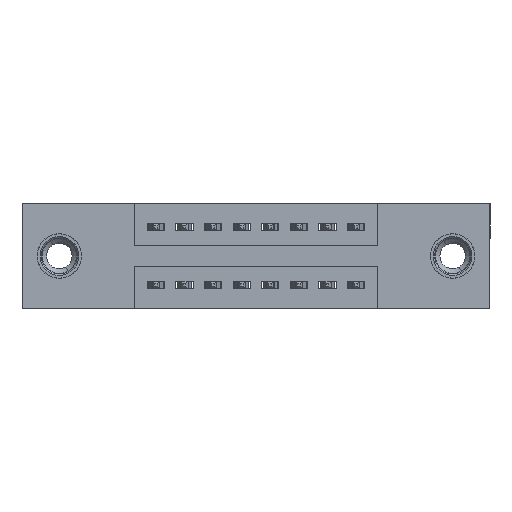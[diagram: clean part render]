
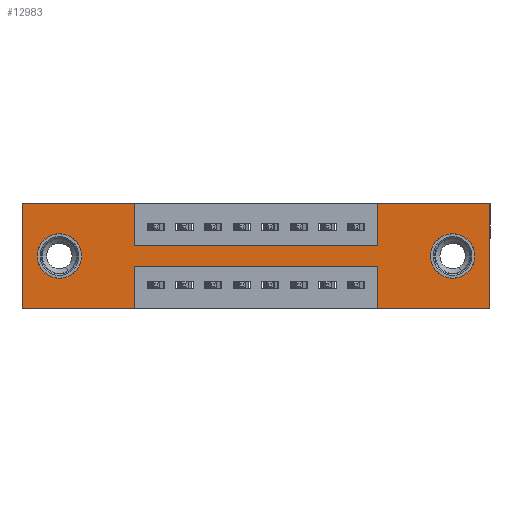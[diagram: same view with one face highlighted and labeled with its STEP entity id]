
A CAD part, front view. The second image highlights one B-rep face of the part: STEP entity #12983.
In plain terms, the highlighted planar face has unit normal (0, -1, 0).
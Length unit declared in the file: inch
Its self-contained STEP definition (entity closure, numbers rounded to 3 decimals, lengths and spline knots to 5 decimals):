
#64 = CARTESIAN_POINT ( 'NONE',  ( 0., 0., 0. ) ) ;
#259 = DIRECTION ( 'NONE',  ( 0., 0., -1. ) ) ;
#395 = VECTOR ( 'NONE', #5062, 39.37008 ) ;
#472 = EDGE_LOOP ( 'NONE', ( #5619, #10605 ) ) ;
#561 = DIRECTION ( 'NONE',  ( 0., 1., 0. ) ) ;
#761 = VERTEX_POINT ( 'NONE', #8621 ) ;
#1044 = CARTESIAN_POINT ( 'NONE',  ( 0.13, 0., -0.107 ) ) ;
#1137 = ORIENTED_EDGE ( 'NONE', *, *, #11477, .F. ) ;
#1145 = ORIENTED_EDGE ( 'NONE', *, *, #5621, .T. ) ;
#1279 = LINE ( 'NONE', #5828, #6372 ) ;
#1359 = EDGE_CURVE ( 'NONE', #10727, #10186, #3395, .T. ) ;
#1416 = VERTEX_POINT ( 'NONE', #9835 ) ;
#1545 = CARTESIAN_POINT ( 'NONE',  ( 1.2425, 0., -0.15 ) ) ;
#1606 = VECTOR ( 'NONE', #2471, 39.37008 ) ;
#1657 = LINE ( 'NONE', #12248, #9697 ) ;
#1683 = AXIS2_PLACEMENT_3D ( 'NONE', #7374, #2345, #9378 ) ;
#1732 = CARTESIAN_POINT ( 'NONE',  ( 0.13, 0., -0.263 ) ) ;
#1822 = CARTESIAN_POINT ( 'NONE',  ( 0., 0., 0. ) ) ;
#1833 = VECTOR ( 'NONE', #11157, 39.37008 ) ;
#1933 = ORIENTED_EDGE ( 'NONE', *, *, #3104, .F. ) ;
#2345 = DIRECTION ( 'NONE',  ( 0., -1., 0. ) ) ;
#2355 = CARTESIAN_POINT ( 'NONE',  ( 1.2425, 0., -0.37 ) ) ;
#2457 = FACE_BOUND ( 'NONE', #6933, .T. ) ;
#2471 = DIRECTION ( 'NONE',  ( -1., 0., 0. ) ) ;
#2588 = ORIENTED_EDGE ( 'NONE', *, *, #7186, .F. ) ;
#2758 = FACE_OUTER_BOUND ( 'NONE', #12592, .T. ) ;
#2913 = CIRCLE ( 'NONE', #12300, 0.078 ) ;
#2937 = CARTESIAN_POINT ( 'NONE',  ( 0.13, 0., -0.185 ) ) ;
#3098 = CIRCLE ( 'NONE', #6126, 0.078 ) ;
#3104 = EDGE_CURVE ( 'NONE', #10186, #7841, #3968, .T. ) ;
#3114 = LINE ( 'NONE', #11016, #395 ) ;
#3244 = LINE ( 'NONE', #5899, #8295 ) ;
#3395 = LINE ( 'NONE', #7033, #8448 ) ;
#3873 = CARTESIAN_POINT ( 'NONE',  ( 1.505, 0., -0.185 ) ) ;
#3944 = DIRECTION ( 'NONE',  ( 0., 0., 1. ) ) ;
#3968 = LINE ( 'NONE', #8499, #1606 ) ;
#4020 = AXIS2_PLACEMENT_3D ( 'NONE', #2937, #9961, #3944 ) ;
#4195 = VECTOR ( 'NONE', #9818, 39.37008 ) ;
#4498 = CARTESIAN_POINT ( 'NONE',  ( 1.2425, 0., -0.22 ) ) ;
#4552 = LINE ( 'NONE', #64, #1833 ) ;
#4839 = DIRECTION ( 'NONE',  ( 0., 0., -1. ) ) ;
#4843 = CARTESIAN_POINT ( 'NONE',  ( 1.635, 0., 0. ) ) ;
#4847 = EDGE_CURVE ( 'NONE', #7894, #5269, #11600, .T. ) ;
#4934 = DIRECTION ( 'NONE',  ( 0., 0., -1. ) ) ;
#5036 = ORIENTED_EDGE ( 'NONE', *, *, #1359, .F. ) ;
#5062 = DIRECTION ( 'NONE',  ( 0., 0., -1. ) ) ;
#5269 = VERTEX_POINT ( 'NONE', #1732 ) ;
#5321 = VERTEX_POINT ( 'NONE', #1822 ) ;
#5619 = ORIENTED_EDGE ( 'NONE', *, *, #4847, .T. ) ;
#5621 = EDGE_CURVE ( 'NONE', #12732, #12567, #8177, .T. ) ;
#5768 = VERTEX_POINT ( 'NONE', #1545 ) ;
#5828 = CARTESIAN_POINT ( 'NONE',  ( 1.2425, 0., -0.37 ) ) ;
#5899 = CARTESIAN_POINT ( 'NONE',  ( 0., 0., 0. ) ) ;
#6044 = CARTESIAN_POINT ( 'NONE',  ( 1.2425, 0., 0. ) ) ;
#6126 = AXIS2_PLACEMENT_3D ( 'NONE', #6665, #561, #7662 ) ;
#6150 = EDGE_CURVE ( 'NONE', #7841, #5321, #4552, .T. ) ;
#6295 = DIRECTION ( 'NONE',  ( -1., 0., 0. ) ) ;
#6366 = DIRECTION ( 'NONE',  ( 0., 1., 0. ) ) ;
#6372 = VECTOR ( 'NONE', #7821, 39.37008 ) ;
#6382 = DIRECTION ( 'NONE',  ( 1., 0., 0. ) ) ;
#6396 = PLANE ( 'NONE',  #1683 ) ;
#6408 = EDGE_CURVE ( 'NONE', #761, #6815, #6458, .T. ) ;
#6458 = LINE ( 'NONE', #10538, #9090 ) ;
#6665 = CARTESIAN_POINT ( 'NONE',  ( 0.13, 0., -0.185 ) ) ;
#6815 = VERTEX_POINT ( 'NONE', #9202 ) ;
#6849 = EDGE_CURVE ( 'NONE', #11630, #8073, #1657, .T. ) ;
#6909 = VECTOR ( 'NONE', #9994, 39.37008 ) ;
#6933 = EDGE_LOOP ( 'NONE', ( #1145, #11306 ) ) ;
#7017 = CARTESIAN_POINT ( 'NONE',  ( 0.3925, 0., -0.22 ) ) ;
#7033 = CARTESIAN_POINT ( 'NONE',  ( 0.3925, 0., -0.37 ) ) ;
#7034 = DIRECTION ( 'NONE',  ( 0., 0., 1. ) ) ;
#7096 = LINE ( 'NONE', #9367, #12402 ) ;
#7186 = EDGE_CURVE ( 'NONE', #5321, #761, #3244, .T. ) ;
#7221 = LINE ( 'NONE', #7017, #6909 ) ;
#7374 = CARTESIAN_POINT ( 'NONE',  ( 0., 0., -0.37 ) ) ;
#7441 = VECTOR ( 'NONE', #7034, 39.37008 ) ;
#7662 = DIRECTION ( 'NONE',  ( 0., 0., 1. ) ) ;
#7667 = ORIENTED_EDGE ( 'NONE', *, *, #11609, .F. ) ;
#7714 = CARTESIAN_POINT ( 'NONE',  ( 0.3925, 0., -0.22 ) ) ;
#7734 = ORIENTED_EDGE ( 'NONE', *, *, #12108, .F. ) ;
#7737 = CARTESIAN_POINT ( 'NONE',  ( 1.505, 0., -0.263 ) ) ;
#7821 = DIRECTION ( 'NONE',  ( 0., 0., 1. ) ) ;
#7841 = VERTEX_POINT ( 'NONE', #9979 ) ;
#7894 = VERTEX_POINT ( 'NONE', #1044 ) ;
#7903 = ORIENTED_EDGE ( 'NONE', *, *, #6408, .F. ) ;
#8016 = CARTESIAN_POINT ( 'NONE',  ( 1.635, 0., -0.37 ) ) ;
#8073 = VERTEX_POINT ( 'NONE', #2355 ) ;
#8177 = CIRCLE ( 'NONE', #10905, 0.078 ) ;
#8295 = VECTOR ( 'NONE', #10808, 39.37008 ) ;
#8448 = VECTOR ( 'NONE', #4839, 39.37008 ) ;
#8499 = CARTESIAN_POINT ( 'NONE',  ( 0., 0., -0.37 ) ) ;
#8560 = DIRECTION ( 'NONE',  ( 0., 0., -1. ) ) ;
#8621 = CARTESIAN_POINT ( 'NONE',  ( 0.3925, 0., 0. ) ) ;
#9090 = VECTOR ( 'NONE', #8560, 39.37008 ) ;
#9202 = CARTESIAN_POINT ( 'NONE',  ( 0.3925, 0., -0.15 ) ) ;
#9367 = CARTESIAN_POINT ( 'NONE',  ( 0.3925, 0., -0.15 ) ) ;
#9378 = DIRECTION ( 'NONE',  ( 0., 0., -1. ) ) ;
#9555 = EDGE_CURVE ( 'NONE', #8073, #11880, #1279, .T. ) ;
#9697 = VECTOR ( 'NONE', #6295, 39.37008 ) ;
#9705 = EDGE_CURVE ( 'NONE', #5768, #1416, #12741, .T. ) ;
#9747 = ORIENTED_EDGE ( 'NONE', *, *, #10442, .F. ) ;
#9782 = CARTESIAN_POINT ( 'NONE',  ( 0., 0., 0. ) ) ;
#9818 = DIRECTION ( 'NONE',  ( 1., 0., 0. ) ) ;
#9835 = CARTESIAN_POINT ( 'NONE',  ( 1.2425, 0., 0. ) ) ;
#9961 = DIRECTION ( 'NONE',  ( 0., 1., 0. ) ) ;
#9979 = CARTESIAN_POINT ( 'NONE',  ( 0., 0., -0.37 ) ) ;
#9994 = DIRECTION ( 'NONE',  ( -1., 0., 0. ) ) ;
#10186 = VERTEX_POINT ( 'NONE', #10913 ) ;
#10364 = ORIENTED_EDGE ( 'NONE', *, *, #6150, .F. ) ;
#10442 = EDGE_CURVE ( 'NONE', #6815, #5768, #7096, .T. ) ;
#10538 = CARTESIAN_POINT ( 'NONE',  ( 0.3925, 0., 0. ) ) ;
#10605 = ORIENTED_EDGE ( 'NONE', *, *, #11965, .T. ) ;
#10727 = VERTEX_POINT ( 'NONE', #7714 ) ;
#10808 = DIRECTION ( 'NONE',  ( 1., 0., 0. ) ) ;
#10882 = DIRECTION ( 'NONE',  ( 0., 1., 0. ) ) ;
#10905 = AXIS2_PLACEMENT_3D ( 'NONE', #12323, #6366, #259 ) ;
#10913 = CARTESIAN_POINT ( 'NONE',  ( 0.3925, 0., -0.37 ) ) ;
#11016 = CARTESIAN_POINT ( 'NONE',  ( 1.635, 0., 0. ) ) ;
#11157 = DIRECTION ( 'NONE',  ( 0., 0., 1. ) ) ;
#11306 = ORIENTED_EDGE ( 'NONE', *, *, #12703, .T. ) ;
#11330 = VERTEX_POINT ( 'NONE', #4843 ) ;
#11477 = EDGE_CURVE ( 'NONE', #11330, #11630, #3114, .T. ) ;
#11600 = CIRCLE ( 'NONE', #4020, 0.078 ) ;
#11609 = EDGE_CURVE ( 'NONE', #11880, #10727, #7221, .T. ) ;
#11630 = VERTEX_POINT ( 'NONE', #8016 ) ;
#11880 = VERTEX_POINT ( 'NONE', #4498 ) ;
#11965 = EDGE_CURVE ( 'NONE', #5269, #7894, #3098, .T. ) ;
#12090 = ORIENTED_EDGE ( 'NONE', *, *, #6849, .F. ) ;
#12108 = EDGE_CURVE ( 'NONE', #1416, #11330, #12205, .T. ) ;
#12205 = LINE ( 'NONE', #9782, #4195 ) ;
#12248 = CARTESIAN_POINT ( 'NONE',  ( 0., 0., -0.37 ) ) ;
#12275 = ORIENTED_EDGE ( 'NONE', *, *, #9705, .F. ) ;
#12300 = AXIS2_PLACEMENT_3D ( 'NONE', #3873, #10882, #4934 ) ;
#12323 = CARTESIAN_POINT ( 'NONE',  ( 1.505, 0., -0.185 ) ) ;
#12402 = VECTOR ( 'NONE', #6382, 39.37008 ) ;
#12567 = VERTEX_POINT ( 'NONE', #7737 ) ;
#12592 = EDGE_LOOP ( 'NONE', ( #5036, #7667, #12992, #12090, #1137, #7734, #12275, #9747, #7903, #2588, #10364, #1933 ) ) ;
#12703 = EDGE_CURVE ( 'NONE', #12567, #12732, #2913, .T. ) ;
#12732 = VERTEX_POINT ( 'NONE', #12957 ) ;
#12741 = LINE ( 'NONE', #6044, #7441 ) ;
#12798 = FACE_BOUND ( 'NONE', #472, .T. ) ;
#12957 = CARTESIAN_POINT ( 'NONE',  ( 1.505, 0., -0.107 ) ) ;
#12983 = ADVANCED_FACE ( 'NONE', ( #2457, #12798, #2758 ), #6396, .T. ) ;
#12992 = ORIENTED_EDGE ( 'NONE', *, *, #9555, .F. ) ;
